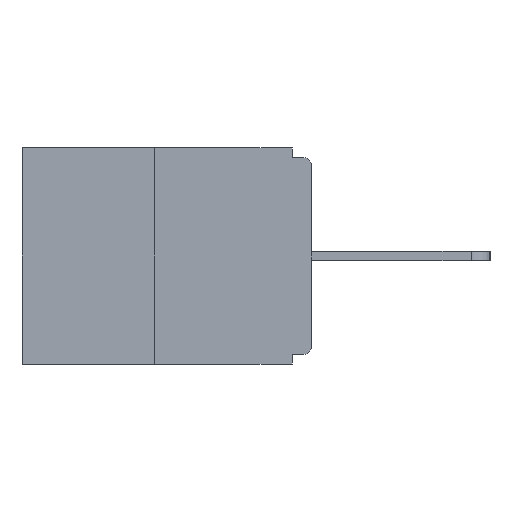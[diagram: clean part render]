
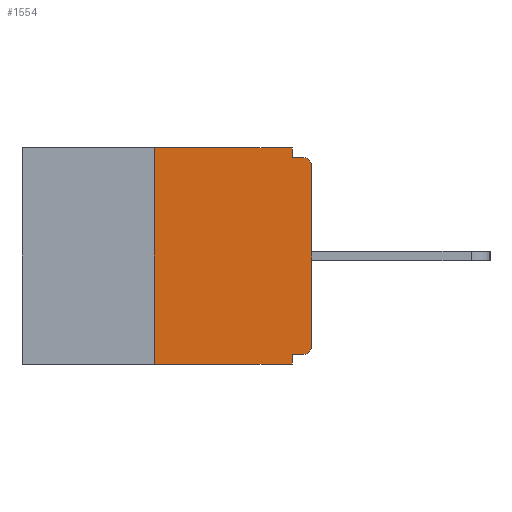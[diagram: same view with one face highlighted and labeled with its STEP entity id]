
A CAD part, left-side view. The second image highlights one B-rep face of the part: STEP entity #1554.
In plain terms, the highlighted planar face has unit normal (-1, 0, 0).
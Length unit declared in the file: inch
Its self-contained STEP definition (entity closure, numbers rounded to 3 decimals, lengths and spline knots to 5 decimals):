
#26 = ORIENTED_EDGE ( 'NONE', *, *, #9883, .F. ) ;
#147 = VECTOR ( 'NONE', #13941, 39.37008 ) ;
#204 = CIRCLE ( 'NONE', #532, 0.015 ) ;
#256 = CARTESIAN_POINT ( 'NONE',  ( 0., 0.031, -0.328 ) ) ;
#532 = AXIS2_PLACEMENT_3D ( 'NONE', #4221, #19068, #13799 ) ;
#1226 = FACE_OUTER_BOUND ( 'NONE', #1252, .T. ) ;
#1252 = EDGE_LOOP ( 'NONE', ( #20405, #11288, #19265, #5307, #26, #10497, #2816, #12633, #10143, #6789 ) ) ;
#1342 = LINE ( 'NONE', #19203, #20520 ) ;
#1554 = ADVANCED_FACE ( 'NONE', ( #1226 ), #15957, .F. ) ;
#1625 = VERTEX_POINT ( 'NONE', #4778 ) ;
#1669 = DIRECTION ( 'NONE',  ( 0., 0., -1. ) ) ;
#1951 = DIRECTION ( 'NONE',  ( 0., 0., -1. ) ) ;
#2695 = VERTEX_POINT ( 'NONE', #3930 ) ;
#2798 = VERTEX_POINT ( 'NONE', #6383 ) ;
#2816 = ORIENTED_EDGE ( 'NONE', *, *, #15854, .T. ) ;
#3367 = CARTESIAN_POINT ( 'NONE',  ( 0., 0.015, -0.015 ) ) ;
#3865 = VECTOR ( 'NONE', #15987, 39.37008 ) ;
#3930 = CARTESIAN_POINT ( 'NONE',  ( 0., 0.031, -0.015 ) ) ;
#4013 = DIRECTION ( 'NONE',  ( 0., 0., 1. ) ) ;
#4221 = CARTESIAN_POINT ( 'NONE',  ( 0., 0.015, -0.313 ) ) ;
#4400 = EDGE_CURVE ( 'NONE', #2798, #18506, #15789, .T. ) ;
#4462 = DIRECTION ( 'NONE',  ( 0., 0., -1. ) ) ;
#4778 = CARTESIAN_POINT ( 'NONE',  ( 0., 0.031, -0.343 ) ) ;
#5307 = ORIENTED_EDGE ( 'NONE', *, *, #9252, .F. ) ;
#6383 = CARTESIAN_POINT ( 'NONE',  ( 0., 0., -0.03 ) ) ;
#6789 = ORIENTED_EDGE ( 'NONE', *, *, #14906, .F. ) ;
#7423 = DIRECTION ( 'NONE',  ( 0., 0., 1. ) ) ;
#7450 = VERTEX_POINT ( 'NONE', #12962 ) ;
#7527 = LINE ( 'NONE', #18841, #11598 ) ;
#7675 = CARTESIAN_POINT ( 'NONE',  ( 0., 0.46, 0. ) ) ;
#8937 = EDGE_CURVE ( 'NONE', #7450, #11963, #9277, .T. ) ;
#8940 = VERTEX_POINT ( 'NONE', #20455 ) ;
#9044 = VECTOR ( 'NONE', #1951, 39.37008 ) ;
#9213 = CARTESIAN_POINT ( 'NONE',  ( 0., 0., -0.015 ) ) ;
#9252 = EDGE_CURVE ( 'NONE', #16982, #1625, #13465, .T. ) ;
#9277 = LINE ( 'NONE', #20258, #21055 ) ;
#9704 = LINE ( 'NONE', #16255, #17687 ) ;
#9883 = EDGE_CURVE ( 'NONE', #8940, #16982, #17604, .T. ) ;
#9965 = CARTESIAN_POINT ( 'NONE',  ( 0., 0.015, -0.03 ) ) ;
#10143 = ORIENTED_EDGE ( 'NONE', *, *, #18966, .F. ) ;
#10497 = ORIENTED_EDGE ( 'NONE', *, *, #19192, .T. ) ;
#11288 = ORIENTED_EDGE ( 'NONE', *, *, #8937, .F. ) ;
#11598 = VECTOR ( 'NONE', #7423, 39.37008 ) ;
#11851 = EDGE_CURVE ( 'NONE', #7450, #1625, #12124, .T. ) ;
#11963 = VERTEX_POINT ( 'NONE', #20936 ) ;
#12124 = LINE ( 'NONE', #18675, #147 ) ;
#12269 = AXIS2_PLACEMENT_3D ( 'NONE', #7675, #17572, #21235 ) ;
#12633 = ORIENTED_EDGE ( 'NONE', *, *, #4400, .T. ) ;
#12962 = CARTESIAN_POINT ( 'NONE',  ( 0., 0.25, -0.343 ) ) ;
#13465 = LINE ( 'NONE', #13568, #9044 ) ;
#13568 = CARTESIAN_POINT ( 'NONE',  ( 0., 0.031, -0.343 ) ) ;
#13799 = DIRECTION ( 'NONE',  ( 0., 0., -1. ) ) ;
#13941 = DIRECTION ( 'NONE',  ( 0., -1., 0. ) ) ;
#14064 = VERTEX_POINT ( 'NONE', #14435 ) ;
#14435 = CARTESIAN_POINT ( 'NONE',  ( 0., 0.031, 0. ) ) ;
#14906 = EDGE_CURVE ( 'NONE', #14064, #2695, #1342, .T. ) ;
#15789 = CIRCLE ( 'NONE', #19239, 0.015 ) ;
#15854 = EDGE_CURVE ( 'NONE', #21066, #2798, #7527, .T. ) ;
#15957 = PLANE ( 'NONE',  #12269 ) ;
#15987 = DIRECTION ( 'NONE',  ( 0., 1., 0. ) ) ;
#16255 = CARTESIAN_POINT ( 'NONE',  ( 0., 0.46, 0. ) ) ;
#16982 = VERTEX_POINT ( 'NONE', #256 ) ;
#17340 = VECTOR ( 'NONE', #19216, 39.37008 ) ;
#17391 = CARTESIAN_POINT ( 'NONE',  ( 0., 0., -0.328 ) ) ;
#17572 = DIRECTION ( 'NONE',  ( 1., 0., 0. ) ) ;
#17604 = LINE ( 'NONE', #17391, #3865 ) ;
#17687 = VECTOR ( 'NONE', #20992, 39.37008 ) ;
#18293 = CARTESIAN_POINT ( 'NONE',  ( 0., 0., -0.313 ) ) ;
#18422 = EDGE_CURVE ( 'NONE', #11963, #14064, #9704, .T. ) ;
#18506 = VERTEX_POINT ( 'NONE', #3367 ) ;
#18675 = CARTESIAN_POINT ( 'NONE',  ( 0., 0.46, -0.343 ) ) ;
#18841 = CARTESIAN_POINT ( 'NONE',  ( 0., 0., 0. ) ) ;
#18966 = EDGE_CURVE ( 'NONE', #2695, #18506, #19321, .T. ) ;
#19068 = DIRECTION ( 'NONE',  ( -1., 0., 0. ) ) ;
#19192 = EDGE_CURVE ( 'NONE', #8940, #21066, #204, .T. ) ;
#19203 = CARTESIAN_POINT ( 'NONE',  ( 0., 0.031, 0. ) ) ;
#19216 = DIRECTION ( 'NONE',  ( 0., -1., 0. ) ) ;
#19239 = AXIS2_PLACEMENT_3D ( 'NONE', #9965, #21245, #1669 ) ;
#19265 = ORIENTED_EDGE ( 'NONE', *, *, #11851, .T. ) ;
#19321 = LINE ( 'NONE', #9213, #17340 ) ;
#20258 = CARTESIAN_POINT ( 'NONE',  ( 0., 0.25, 0. ) ) ;
#20405 = ORIENTED_EDGE ( 'NONE', *, *, #18422, .F. ) ;
#20455 = CARTESIAN_POINT ( 'NONE',  ( 0., 0.015, -0.328 ) ) ;
#20520 = VECTOR ( 'NONE', #4462, 39.37008 ) ;
#20936 = CARTESIAN_POINT ( 'NONE',  ( 0., 0.25, 0. ) ) ;
#20992 = DIRECTION ( 'NONE',  ( 0., -1., 0. ) ) ;
#21055 = VECTOR ( 'NONE', #4013, 39.37008 ) ;
#21066 = VERTEX_POINT ( 'NONE', #18293 ) ;
#21235 = DIRECTION ( 'NONE',  ( 0., 0., -1. ) ) ;
#21245 = DIRECTION ( 'NONE',  ( -1., 0., 0. ) ) ;
